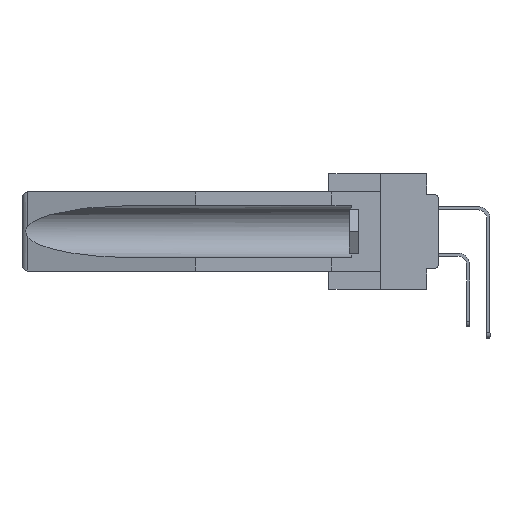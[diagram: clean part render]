
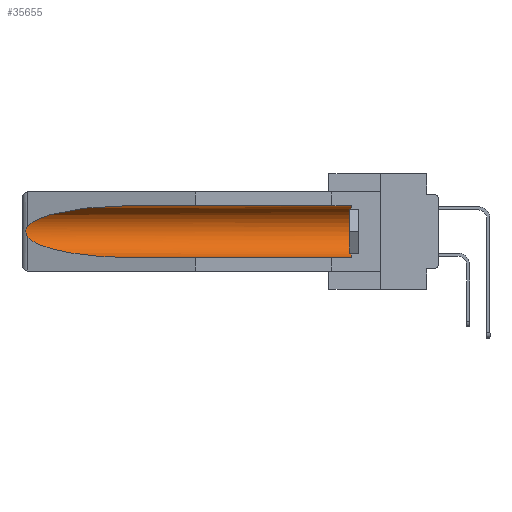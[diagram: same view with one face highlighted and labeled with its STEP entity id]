
A CAD part, left-side view. The second image highlights one B-rep face of the part: STEP entity #35655.
In plain terms, the highlighted cylindrical face has radius 2.857 mm (diameter 5.715 mm), a partial arc.
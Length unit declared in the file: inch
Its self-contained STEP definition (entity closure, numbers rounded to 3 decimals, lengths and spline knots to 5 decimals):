
#14 = EDGE_CURVE ( 'NONE', #564, #8322, #21144, .T. ) ;
#324 = CARTESIAN_POINT ( 'NONE',  ( 0.155, 1.07973, -0.059 ) ) ;
#564 = VERTEX_POINT ( 'NONE', #9249 ) ;
#1128 = ORIENTED_EDGE ( 'NONE', *, *, #17368, .T. ) ;
#1574 = ORIENTED_EDGE ( 'NONE', *, *, #6655, .T. ) ;
#1701 = CYLINDRICAL_SURFACE ( 'NONE', #32404, 0.1125 ) ;
#2078 = DIRECTION ( 'NONE',  ( 0., 1., 0. ) ) ;
#3583 = AXIS2_PLACEMENT_3D ( 'NONE', #18499, #13382, #18686 ) ;
#3646 = CARTESIAN_POINT ( 'NONE',  ( 0.26537, 1.52718, -0.14972 ) ) ;
#3675 = EDGE_CURVE ( 'NONE', #30671, #18075, #36952, .T. ) ;
#4257 = DIRECTION ( 'NONE',  ( 0., 1., 0. ) ) ;
#4445 = CARTESIAN_POINT ( 'NONE',  ( 0.155, -0.30754, -0.059 ) ) ;
#6655 = EDGE_CURVE ( 'NONE', #35819, #21403, #19933, .T. ) ;
#6801 = EDGE_CURVE ( 'NONE', #35819, #8322, #23350, .T. ) ;
#6869 = CARTESIAN_POINT ( 'NONE',  ( 0.26597, 1.52961, -0.15275 ) ) ;
#7790 = ORIENTED_EDGE ( 'NONE', *, *, #16394, .T. ) ;
#8322 = VERTEX_POINT ( 'NONE', #18083 ) ;
#9152 = CARTESIAN_POINT ( 'NONE',  ( 0.26654, 1.53092, -0.15636 ) ) ;
#9249 = CARTESIAN_POINT ( 'NONE',  ( 0.26537, 1.52718, -0.19328 ) ) ;
#9641 = CARTESIAN_POINT ( 'NONE',  ( 0.155, 0.126, -0.284 ) ) ;
#10534 = B_SPLINE_CURVE_WITH_KNOTS ( 'NONE', 3,
 ( #3646, #6869, #9152, #26225, #20904, #20727, #18248, #24120, #14853, #18436 ),
 .UNSPECIFIED., .F., .F.,
 ( 4, 2, 2, 2, 4 ),
 ( 0., 0.00029, 0.00058, 0.00087, 0.00117 ),
 .UNSPECIFIED. ) ;
#12050 = CARTESIAN_POINT ( 'NONE',  ( 0.25451, 1.48313, -0.09465 ) ) ;
#12111 = ORIENTED_EDGE ( 'NONE', *, *, #6801, .F. ) ;
#13382 = DIRECTION ( 'NONE',  ( 0., -1., 0. ) ) ;
#13825 = FACE_OUTER_BOUND ( 'NONE', #32748, .T. ) ;
#14853 = CARTESIAN_POINT ( 'NONE',  ( 0.26597, 1.5296, -0.19026 ) ) ;
#16394 = EDGE_CURVE ( 'NONE', #18075, #564, #10534, .T. ) ;
#17368 = EDGE_CURVE ( 'NONE', #21403, #30671, #27768, .T. ) ;
#18075 = VERTEX_POINT ( 'NONE', #36825 ) ;
#18083 = CARTESIAN_POINT ( 'NONE',  ( 0.155, 1.07973, -0.284 ) ) ;
#18248 = CARTESIAN_POINT ( 'NONE',  ( 0.2673, 1.53269, -0.17917 ) ) ;
#18436 = CARTESIAN_POINT ( 'NONE',  ( 0.26537, 1.52718, -0.19328 ) ) ;
#18499 = CARTESIAN_POINT ( 'NONE',  ( 0.155, 0.126, -0.1715 ) ) ;
#18686 = DIRECTION ( 'NONE',  ( 0., 0., 1. ) ) ;
#19933 = CIRCLE ( 'NONE', #3583, 0.1125 ) ;
#20295 = CARTESIAN_POINT ( 'NONE',  ( 0.21114, 1.30732, -0.284 ) ) ;
#20318 = DIRECTION ( 'NONE',  ( 0., 1., 0. ) ) ;
#20727 = CARTESIAN_POINT ( 'NONE',  ( 0.2675, 1.53308, -0.17534 ) ) ;
#20904 = CARTESIAN_POINT ( 'NONE',  ( 0.2675, 1.53308, -0.16763 ) ) ;
#21144 =( BOUNDED_CURVE ( )  B_SPLINE_CURVE ( 3, ( #29028, #28271, #20295, #34358 ),
 .UNSPECIFIED., .F., .F. ) 
 B_SPLINE_CURVE_WITH_KNOTS ( ( 4, 4 ),
 ( 0.1948, 1.5708 ),
 .UNSPECIFIED. ) 
 CURVE ( )  GEOMETRIC_REPRESENTATION_ITEM ( )  RATIONAL_B_SPLINE_CURVE ( ( 1., 0.848, 0.848, 1. ) ) 
 REPRESENTATION_ITEM ( '' )  );
#21403 = VERTEX_POINT ( 'NONE', #22256 ) ;
#21656 = VECTOR ( 'NONE', #4257, 39.37008 ) ;
#21989 = CARTESIAN_POINT ( 'NONE',  ( 0.155, -0.30754, -0.1715 ) ) ;
#22256 = CARTESIAN_POINT ( 'NONE',  ( 0.155, 0.126, -0.059 ) ) ;
#23350 = LINE ( 'NONE', #33860, #23565 ) ;
#23565 = VECTOR ( 'NONE', #20318, 39.37008 ) ;
#24120 = CARTESIAN_POINT ( 'NONE',  ( 0.26655, 1.53094, -0.18657 ) ) ;
#26225 = CARTESIAN_POINT ( 'NONE',  ( 0.2673, 1.5327, -0.16383 ) ) ;
#27519 = CARTESIAN_POINT ( 'NONE',  ( 0.155, 1.07973, -0.059 ) ) ;
#27768 = LINE ( 'NONE', #4445, #21656 ) ;
#28015 = ORIENTED_EDGE ( 'NONE', *, *, #14, .T. ) ;
#28097 = ORIENTED_EDGE ( 'NONE', *, *, #3675, .T. ) ;
#28271 = CARTESIAN_POINT ( 'NONE',  ( 0.25451, 1.48313, -0.24835 ) ) ;
#28409 = DIRECTION ( 'NONE',  ( 0., 0., 1. ) ) ;
#29028 = CARTESIAN_POINT ( 'NONE',  ( 0.26537, 1.52718, -0.19328 ) ) ;
#29885 = CARTESIAN_POINT ( 'NONE',  ( 0.26537, 1.52718, -0.14972 ) ) ;
#30671 = VERTEX_POINT ( 'NONE', #27519 ) ;
#32404 = AXIS2_PLACEMENT_3D ( 'NONE', #21989, #2078, #28409 ) ;
#32748 = EDGE_LOOP ( 'NONE', ( #28097, #7790, #28015, #12111, #1574, #1128 ) ) ;
#33860 = CARTESIAN_POINT ( 'NONE',  ( 0.155, -0.30754, -0.284 ) ) ;
#34358 = CARTESIAN_POINT ( 'NONE',  ( 0.155, 1.07973, -0.284 ) ) ;
#35002 = CARTESIAN_POINT ( 'NONE',  ( 0.21114, 1.30732, -0.059 ) ) ;
#35655 = ADVANCED_FACE ( 'NONE', ( #13825 ), #1701, .F. ) ;
#35819 = VERTEX_POINT ( 'NONE', #9641 ) ;
#36825 = CARTESIAN_POINT ( 'NONE',  ( 0.26537, 1.52718, -0.14972 ) ) ;
#36952 =( BOUNDED_CURVE ( )  B_SPLINE_CURVE ( 3, ( #324, #35002, #12050, #29885 ),
 .UNSPECIFIED., .F., .F. ) 
 B_SPLINE_CURVE_WITH_KNOTS ( ( 4, 4 ),
 ( 4.71239, 6.08839 ),
 .UNSPECIFIED. ) 
 CURVE ( )  GEOMETRIC_REPRESENTATION_ITEM ( )  RATIONAL_B_SPLINE_CURVE ( ( 1., 0.848, 0.848, 1. ) ) 
 REPRESENTATION_ITEM ( '' )  );
